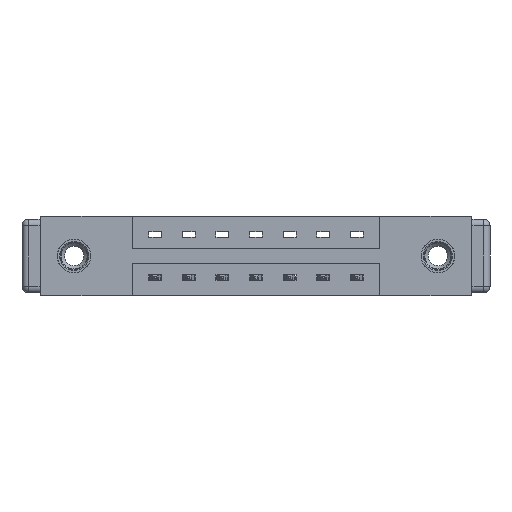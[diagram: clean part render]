
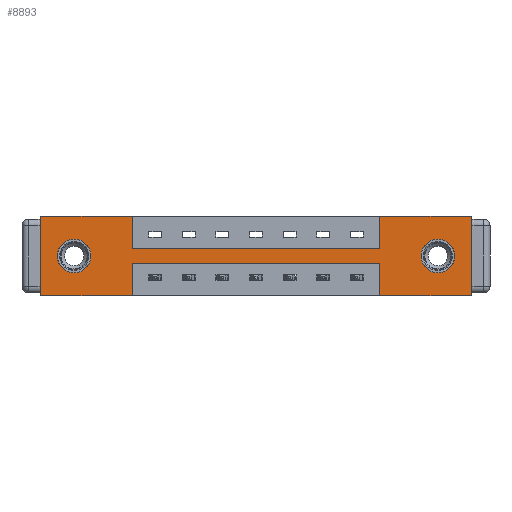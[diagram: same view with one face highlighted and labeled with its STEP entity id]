
A CAD part, front view. The second image highlights one B-rep face of the part: STEP entity #8893.
In plain terms, the highlighted planar face has unit normal (0, -1, 0).
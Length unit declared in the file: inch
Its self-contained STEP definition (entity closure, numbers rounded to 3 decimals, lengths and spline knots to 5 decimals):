
#14 = AXIS2_PLACEMENT_3D ( 'NONE', #6883, #8822, #11625 ) ;
#99 = ORIENTED_EDGE ( 'NONE', *, *, #10944, .F. ) ;
#160 = DIRECTION ( 'NONE',  ( 1., 0., 0. ) ) ;
#246 = VERTEX_POINT ( 'NONE', #9360 ) ;
#253 = VECTOR ( 'NONE', #7765, 39.37008 ) ;
#351 = LINE ( 'NONE', #6216, #8417 ) ;
#380 = EDGE_CURVE ( 'NONE', #3195, #1396, #7323, .T. ) ;
#390 = VERTEX_POINT ( 'NONE', #6699 ) ;
#456 = VECTOR ( 'NONE', #12076, 39.37008 ) ;
#586 = ORIENTED_EDGE ( 'NONE', *, *, #9421, .F. ) ;
#772 = CARTESIAN_POINT ( 'NONE',  ( 1.843, 0., -0.107 ) ) ;
#800 = ORIENTED_EDGE ( 'NONE', *, *, #2616, .T. ) ;
#900 = CARTESIAN_POINT ( 'NONE',  ( 0.155, 0., -0.185 ) ) ;
#987 = CARTESIAN_POINT ( 'NONE',  ( 1.573, 0., -0.37 ) ) ;
#1351 = CARTESIAN_POINT ( 'NONE',  ( 0.425, 0., -0.37 ) ) ;
#1396 = VERTEX_POINT ( 'NONE', #9250 ) ;
#1406 = CARTESIAN_POINT ( 'NONE',  ( 1.998, 0., -0.37 ) ) ;
#1528 = DIRECTION ( 'NONE',  ( 0., 0., 1. ) ) ;
#1751 = VERTEX_POINT ( 'NONE', #9636 ) ;
#2074 = ORIENTED_EDGE ( 'NONE', *, *, #4665, .F. ) ;
#2227 = ORIENTED_EDGE ( 'NONE', *, *, #5095, .F. ) ;
#2397 = DIRECTION ( 'NONE',  ( 0., 0., 1. ) ) ;
#2523 = ORIENTED_EDGE ( 'NONE', *, *, #10139, .T. ) ;
#2616 = EDGE_CURVE ( 'NONE', #8141, #1751, #12065, .T. ) ;
#2621 = ORIENTED_EDGE ( 'NONE', *, *, #380, .F. ) ;
#2658 = CARTESIAN_POINT ( 'NONE',  ( 0., 0., 0. ) ) ;
#2681 = DIRECTION ( 'NONE',  ( 0., 0., -1. ) ) ;
#3165 = EDGE_CURVE ( 'NONE', #11825, #10499, #9830, .T. ) ;
#3195 = VERTEX_POINT ( 'NONE', #10481 ) ;
#3277 = LINE ( 'NONE', #3378, #10763 ) ;
#3352 = EDGE_CURVE ( 'NONE', #9099, #246, #3681, .T. ) ;
#3378 = CARTESIAN_POINT ( 'NONE',  ( 0., 0., -0.37 ) ) ;
#3606 = ORIENTED_EDGE ( 'NONE', *, *, #3746, .T. ) ;
#3635 = FACE_OUTER_BOUND ( 'NONE', #8064, .T. ) ;
#3681 = LINE ( 'NONE', #1351, #9068 ) ;
#3725 = CARTESIAN_POINT ( 'NONE',  ( 0., 0., 0. ) ) ;
#3746 = EDGE_CURVE ( 'NONE', #7953, #10573, #11467, .T. ) ;
#3751 = LINE ( 'NONE', #5234, #8687 ) ;
#3919 = DIRECTION ( 'NONE',  ( 0., 0., -1. ) ) ;
#3937 = LINE ( 'NONE', #10797, #4086 ) ;
#3955 = EDGE_CURVE ( 'NONE', #390, #3195, #9685, .T. ) ;
#4086 = VECTOR ( 'NONE', #160, 39.37008 ) ;
#4114 = VERTEX_POINT ( 'NONE', #9700 ) ;
#4336 = DIRECTION ( 'NONE',  ( 0., -1., 0. ) ) ;
#4358 = AXIS2_PLACEMENT_3D ( 'NONE', #8769, #10684, #5353 ) ;
#4448 = CARTESIAN_POINT ( 'NONE',  ( 0.425, 0., 0. ) ) ;
#4612 = EDGE_LOOP ( 'NONE', ( #3606, #11774 ) ) ;
#4665 = EDGE_CURVE ( 'NONE', #5890, #11825, #8360, .T. ) ;
#4960 = CARTESIAN_POINT ( 'NONE',  ( 1.573, 0., -0.22 ) ) ;
#4982 = LINE ( 'NONE', #9364, #9762 ) ;
#5026 = VERTEX_POINT ( 'NONE', #7169 ) ;
#5090 = LINE ( 'NONE', #6444, #6031 ) ;
#5095 = EDGE_CURVE ( 'NONE', #246, #4114, #3277, .T. ) ;
#5177 = ORIENTED_EDGE ( 'NONE', *, *, #8004, .F. ) ;
#5234 = CARTESIAN_POINT ( 'NONE',  ( 1.573, 0., 0. ) ) ;
#5353 = DIRECTION ( 'NONE',  ( 0., 0., 1. ) ) ;
#5470 = CIRCLE ( 'NONE', #8041, 0.078 ) ;
#5576 = CARTESIAN_POINT ( 'NONE',  ( 1.573, 0., 0. ) ) ;
#5667 = CARTESIAN_POINT ( 'NONE',  ( 0.425, 0., -0.15 ) ) ;
#5844 = DIRECTION ( 'NONE',  ( 0., 1., 0. ) ) ;
#5890 = VERTEX_POINT ( 'NONE', #1406 ) ;
#6031 = VECTOR ( 'NONE', #10196, 39.37008 ) ;
#6216 = CARTESIAN_POINT ( 'NONE',  ( 1.998, 0., 0. ) ) ;
#6218 = EDGE_LOOP ( 'NONE', ( #800, #2523 ) ) ;
#6245 = ORIENTED_EDGE ( 'NONE', *, *, #10487, .F. ) ;
#6392 = PLANE ( 'NONE',  #8550 ) ;
#6444 = CARTESIAN_POINT ( 'NONE',  ( 0., 0., 0. ) ) ;
#6645 = CARTESIAN_POINT ( 'NONE',  ( 1.573, 0., -0.37 ) ) ;
#6699 = CARTESIAN_POINT ( 'NONE',  ( 0.425, 0., 0. ) ) ;
#6883 = CARTESIAN_POINT ( 'NONE',  ( 1.843, 0., -0.185 ) ) ;
#6999 = CIRCLE ( 'NONE', #14, 0.078 ) ;
#7039 = DIRECTION ( 'NONE',  ( 0., 1., 0. ) ) ;
#7080 = DIRECTION ( 'NONE',  ( 0., 0., 1. ) ) ;
#7169 = CARTESIAN_POINT ( 'NONE',  ( 1.998, 0., 0. ) ) ;
#7323 = LINE ( 'NONE', #5667, #12137 ) ;
#7341 = VERTEX_POINT ( 'NONE', #5576 ) ;
#7529 = DIRECTION ( 'NONE',  ( 1., 0., 0. ) ) ;
#7765 = DIRECTION ( 'NONE',  ( 0., 0., 1. ) ) ;
#7953 = VERTEX_POINT ( 'NONE', #8532 ) ;
#8004 = EDGE_CURVE ( 'NONE', #4114, #11828, #10073, .T. ) ;
#8041 = AXIS2_PLACEMENT_3D ( 'NONE', #900, #7039, #7080 ) ;
#8064 = EDGE_LOOP ( 'NONE', ( #8119, #9943, #11752, #2074, #12151, #99, #6245, #2621, #8106, #586, #5177, #2227 ) ) ;
#8106 = ORIENTED_EDGE ( 'NONE', *, *, #3955, .F. ) ;
#8119 = ORIENTED_EDGE ( 'NONE', *, *, #3352, .F. ) ;
#8141 = VERTEX_POINT ( 'NONE', #772 ) ;
#8192 = DIRECTION ( 'NONE',  ( -1., 0., 0. ) ) ;
#8212 = DIRECTION ( 'NONE',  ( 0., 0., -1. ) ) ;
#8271 = EDGE_CURVE ( 'NONE', #10573, #7953, #5470, .T. ) ;
#8360 = LINE ( 'NONE', #11205, #456 ) ;
#8417 = VECTOR ( 'NONE', #11157, 39.37008 ) ;
#8485 = DIRECTION ( 'NONE',  ( -1., 0., 0. ) ) ;
#8532 = CARTESIAN_POINT ( 'NONE',  ( 0.155, 0., -0.107 ) ) ;
#8550 = AXIS2_PLACEMENT_3D ( 'NONE', #12066, #4336, #8212 ) ;
#8687 = VECTOR ( 'NONE', #2397, 39.37008 ) ;
#8769 = CARTESIAN_POINT ( 'NONE',  ( 0.155, 0., -0.185 ) ) ;
#8822 = DIRECTION ( 'NONE',  ( 0., 1., 0. ) ) ;
#8893 = ADVANCED_FACE ( 'NONE', ( #11400, #10813, #3635 ), #6392, .T. ) ;
#8932 = EDGE_CURVE ( 'NONE', #5026, #5890, #351, .T. ) ;
#9068 = VECTOR ( 'NONE', #11127, 39.37008 ) ;
#9099 = VERTEX_POINT ( 'NONE', #9586 ) ;
#9250 = CARTESIAN_POINT ( 'NONE',  ( 1.573, 0., -0.15 ) ) ;
#9360 = CARTESIAN_POINT ( 'NONE',  ( 0.425, 0., -0.37 ) ) ;
#9364 = CARTESIAN_POINT ( 'NONE',  ( 0.425, 0., -0.22 ) ) ;
#9369 = VECTOR ( 'NONE', #2681, 39.37008 ) ;
#9421 = EDGE_CURVE ( 'NONE', #11828, #390, #3937, .T. ) ;
#9586 = CARTESIAN_POINT ( 'NONE',  ( 0.425, 0., -0.22 ) ) ;
#9636 = CARTESIAN_POINT ( 'NONE',  ( 1.843, 0., -0.263 ) ) ;
#9685 = LINE ( 'NONE', #4448, #9369 ) ;
#9700 = CARTESIAN_POINT ( 'NONE',  ( 0., 0., -0.37 ) ) ;
#9760 = EDGE_CURVE ( 'NONE', #10499, #9099, #4982, .T. ) ;
#9762 = VECTOR ( 'NONE', #8485, 39.37008 ) ;
#9830 = LINE ( 'NONE', #6645, #253 ) ;
#9943 = ORIENTED_EDGE ( 'NONE', *, *, #9760, .F. ) ;
#10073 = LINE ( 'NONE', #2658, #11717 ) ;
#10139 = EDGE_CURVE ( 'NONE', #1751, #8141, #6999, .T. ) ;
#10196 = DIRECTION ( 'NONE',  ( 1., 0., 0. ) ) ;
#10481 = CARTESIAN_POINT ( 'NONE',  ( 0.425, 0., -0.15 ) ) ;
#10487 = EDGE_CURVE ( 'NONE', #1396, #7341, #3751, .T. ) ;
#10499 = VERTEX_POINT ( 'NONE', #4960 ) ;
#10573 = VERTEX_POINT ( 'NONE', #11259 ) ;
#10684 = DIRECTION ( 'NONE',  ( 0., 1., 0. ) ) ;
#10763 = VECTOR ( 'NONE', #8192, 39.37008 ) ;
#10797 = CARTESIAN_POINT ( 'NONE',  ( 0., 0., 0. ) ) ;
#10813 = FACE_BOUND ( 'NONE', #4612, .T. ) ;
#10944 = EDGE_CURVE ( 'NONE', #7341, #5026, #5090, .T. ) ;
#11127 = DIRECTION ( 'NONE',  ( 0., 0., -1. ) ) ;
#11147 = AXIS2_PLACEMENT_3D ( 'NONE', #11668, #5844, #3919 ) ;
#11157 = DIRECTION ( 'NONE',  ( 0., 0., -1. ) ) ;
#11205 = CARTESIAN_POINT ( 'NONE',  ( 0., 0., -0.37 ) ) ;
#11259 = CARTESIAN_POINT ( 'NONE',  ( 0.155, 0., -0.263 ) ) ;
#11400 = FACE_BOUND ( 'NONE', #6218, .T. ) ;
#11467 = CIRCLE ( 'NONE', #4358, 0.078 ) ;
#11625 = DIRECTION ( 'NONE',  ( 0., 0., -1. ) ) ;
#11668 = CARTESIAN_POINT ( 'NONE',  ( 1.843, 0., -0.185 ) ) ;
#11717 = VECTOR ( 'NONE', #1528, 39.37008 ) ;
#11752 = ORIENTED_EDGE ( 'NONE', *, *, #3165, .F. ) ;
#11774 = ORIENTED_EDGE ( 'NONE', *, *, #8271, .T. ) ;
#11825 = VERTEX_POINT ( 'NONE', #987 ) ;
#11828 = VERTEX_POINT ( 'NONE', #3725 ) ;
#12065 = CIRCLE ( 'NONE', #11147, 0.078 ) ;
#12066 = CARTESIAN_POINT ( 'NONE',  ( 0., 0., -0.37 ) ) ;
#12076 = DIRECTION ( 'NONE',  ( -1., 0., 0. ) ) ;
#12137 = VECTOR ( 'NONE', #7529, 39.37008 ) ;
#12151 = ORIENTED_EDGE ( 'NONE', *, *, #8932, .F. ) ;
